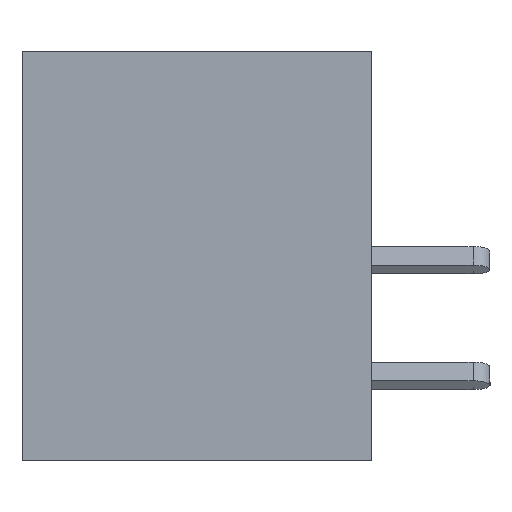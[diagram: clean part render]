
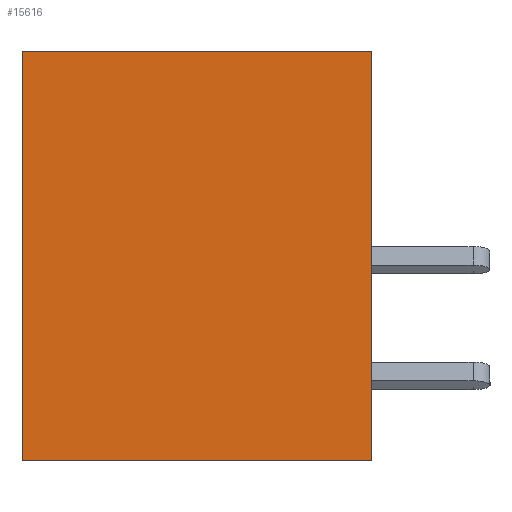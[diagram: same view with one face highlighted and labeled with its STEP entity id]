
A CAD part, left-side view. The second image highlights one B-rep face of the part: STEP entity #15616.
In plain terms, the highlighted planar face has unit normal (-1, 0, 0).
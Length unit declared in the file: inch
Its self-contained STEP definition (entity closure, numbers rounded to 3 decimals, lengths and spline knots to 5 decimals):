
#561 = CARTESIAN_POINT ( 'NONE',  ( 0., 0., 0. ) ) ;
#807 = LINE ( 'NONE', #23656, #12555 ) ;
#1339 = CARTESIAN_POINT ( 'NONE',  ( 0., 0.453, 0. ) ) ;
#2158 = VERTEX_POINT ( 'NONE', #561 ) ;
#4575 = EDGE_CURVE ( 'NONE', #18284, #23122, #14346, .T. ) ;
#6289 = VECTOR ( 'NONE', #16754, 39.37008 ) ;
#7582 = EDGE_CURVE ( 'NONE', #18284, #13111, #8348, .T. ) ;
#7741 = AXIS2_PLACEMENT_3D ( 'NONE', #1339, #8903, #10853 ) ;
#8348 = LINE ( 'NONE', #14890, #6289 ) ;
#8903 = DIRECTION ( 'NONE',  ( 1., 0., 0. ) ) ;
#8980 = PLANE ( 'NONE',  #7741 ) ;
#9004 = ORIENTED_EDGE ( 'NONE', *, *, #17099, .T. ) ;
#9495 = CARTESIAN_POINT ( 'NONE',  ( 0., 0., -0.531 ) ) ;
#9733 = DIRECTION ( 'NONE',  ( 0., 0., 1. ) ) ;
#9877 = LINE ( 'NONE', #21405, #20445 ) ;
#10853 = DIRECTION ( 'NONE',  ( 0., 0., -1. ) ) ;
#11774 = EDGE_LOOP ( 'NONE', ( #9004, #14875, #14636, #24229 ) ) ;
#12555 = VECTOR ( 'NONE', #14179, 39.37008 ) ;
#13111 = VERTEX_POINT ( 'NONE', #9495 ) ;
#13837 = DIRECTION ( 'NONE',  ( 0., -1., 0. ) ) ;
#14179 = DIRECTION ( 'NONE',  ( 0., 0., 1. ) ) ;
#14296 = CARTESIAN_POINT ( 'NONE',  ( 0., 0.453, -0.531 ) ) ;
#14346 = LINE ( 'NONE', #20960, #18448 ) ;
#14636 = ORIENTED_EDGE ( 'NONE', *, *, #4575, .F. ) ;
#14875 = ORIENTED_EDGE ( 'NONE', *, *, #17703, .F. ) ;
#14890 = CARTESIAN_POINT ( 'NONE',  ( 0., 0.453, -0.531 ) ) ;
#15616 = ADVANCED_FACE ( 'NONE', ( #20866 ), #8980, .F. ) ;
#16754 = DIRECTION ( 'NONE',  ( 0., -1., 0. ) ) ;
#17099 = EDGE_CURVE ( 'NONE', #13111, #2158, #807, .T. ) ;
#17472 = CARTESIAN_POINT ( 'NONE',  ( 0., 0.453, 0. ) ) ;
#17703 = EDGE_CURVE ( 'NONE', #23122, #2158, #9877, .T. ) ;
#18284 = VERTEX_POINT ( 'NONE', #14296 ) ;
#18448 = VECTOR ( 'NONE', #9733, 39.37008 ) ;
#20445 = VECTOR ( 'NONE', #13837, 39.37008 ) ;
#20866 = FACE_OUTER_BOUND ( 'NONE', #11774, .T. ) ;
#20960 = CARTESIAN_POINT ( 'NONE',  ( 0., 0.453, 0. ) ) ;
#21405 = CARTESIAN_POINT ( 'NONE',  ( 0., 0.453, 0. ) ) ;
#23122 = VERTEX_POINT ( 'NONE', #17472 ) ;
#23656 = CARTESIAN_POINT ( 'NONE',  ( 0., 0., 0. ) ) ;
#24229 = ORIENTED_EDGE ( 'NONE', *, *, #7582, .T. ) ;
